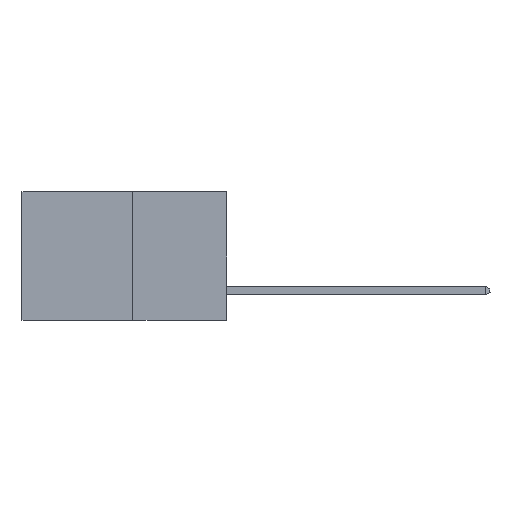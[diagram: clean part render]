
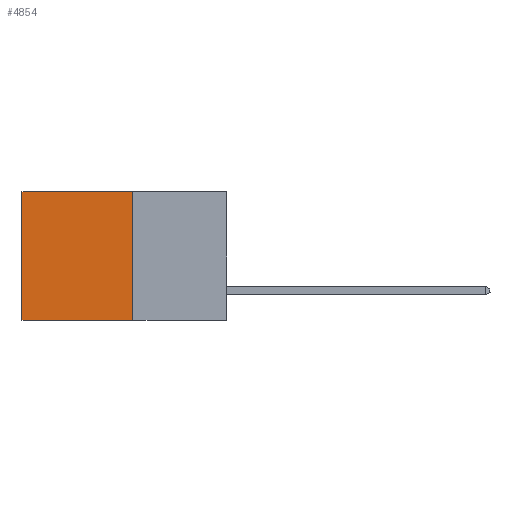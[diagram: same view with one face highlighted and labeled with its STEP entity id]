
A CAD part, left-side view. The second image highlights one B-rep face of the part: STEP entity #4854.
In plain terms, the highlighted planar face has unit normal (-1, 0, 0).
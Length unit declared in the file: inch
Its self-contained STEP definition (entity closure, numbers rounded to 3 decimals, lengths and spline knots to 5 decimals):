
#18 = CARTESIAN_POINT ( 'NONE',  ( 0.277, 0.27, 0. ) ) ;
#374 = ORIENTED_EDGE ( 'NONE', *, *, #899, .F. ) ;
#376 = EDGE_CURVE ( 'NONE', #3596, #5632, #5226, .T. ) ;
#899 = EDGE_CURVE ( 'NONE', #3417, #3596, #8948, .T. ) ;
#1662 = VECTOR ( 'NONE', #7000, 39.37008 ) ;
#2057 = DIRECTION ( 'NONE',  ( 0., 1., 0. ) ) ;
#2219 = VECTOR ( 'NONE', #5075, 39.37008 ) ;
#2399 = EDGE_LOOP ( 'NONE', ( #8888, #3558, #374, #8772 ) ) ;
#2473 = LINE ( 'NONE', #18, #2219 ) ;
#2838 = CARTESIAN_POINT ( 'NONE',  ( 0.277, 0.27, -0.37 ) ) ;
#3005 = CARTESIAN_POINT ( 'NONE',  ( 0.277, 0.59, -0.37 ) ) ;
#3417 = VERTEX_POINT ( 'NONE', #8185 ) ;
#3558 = ORIENTED_EDGE ( 'NONE', *, *, #376, .F. ) ;
#3596 = VERTEX_POINT ( 'NONE', #7999 ) ;
#4063 = LINE ( 'NONE', #6982, #1662 ) ;
#4438 = CARTESIAN_POINT ( 'NONE',  ( 0.277, 0.27, -0.37 ) ) ;
#4642 = CARTESIAN_POINT ( 'NONE',  ( 0.277, 0.59, 0. ) ) ;
#4853 = AXIS2_PLACEMENT_3D ( 'NONE', #9558, #9777, #9594 ) ;
#4854 = ADVANCED_FACE ( 'NONE', ( #8963 ), #9140, .F. ) ;
#4967 = VECTOR ( 'NONE', #7335, 39.37008 ) ;
#4981 = VECTOR ( 'NONE', #2057, 39.37008 ) ;
#5075 = DIRECTION ( 'NONE',  ( 0., 1., 0. ) ) ;
#5226 = LINE ( 'NONE', #2838, #4981 ) ;
#5507 = VERTEX_POINT ( 'NONE', #4642 ) ;
#5632 = VERTEX_POINT ( 'NONE', #3005 ) ;
#6557 = EDGE_CURVE ( 'NONE', #5507, #5632, #4063, .T. ) ;
#6982 = CARTESIAN_POINT ( 'NONE',  ( 0.277, 0.59, -0.37 ) ) ;
#7000 = DIRECTION ( 'NONE',  ( 0., 0., -1. ) ) ;
#7335 = DIRECTION ( 'NONE',  ( 0., 0., -1. ) ) ;
#7999 = CARTESIAN_POINT ( 'NONE',  ( 0.277, 0.27, -0.37 ) ) ;
#8185 = CARTESIAN_POINT ( 'NONE',  ( 0.277, 0.27, 0. ) ) ;
#8772 = ORIENTED_EDGE ( 'NONE', *, *, #9542, .T. ) ;
#8888 = ORIENTED_EDGE ( 'NONE', *, *, #6557, .T. ) ;
#8948 = LINE ( 'NONE', #4438, #4967 ) ;
#8963 = FACE_OUTER_BOUND ( 'NONE', #2399, .T. ) ;
#9140 = PLANE ( 'NONE',  #4853 ) ;
#9542 = EDGE_CURVE ( 'NONE', #3417, #5507, #2473, .T. ) ;
#9558 = CARTESIAN_POINT ( 'NONE',  ( 0.277, 0.27, -0.37 ) ) ;
#9594 = DIRECTION ( 'NONE',  ( 0., 0., -1. ) ) ;
#9777 = DIRECTION ( 'NONE',  ( 1., 0., 0. ) ) ;
